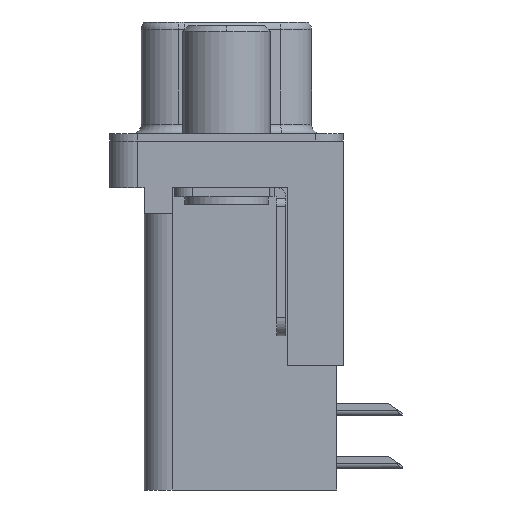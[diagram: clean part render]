
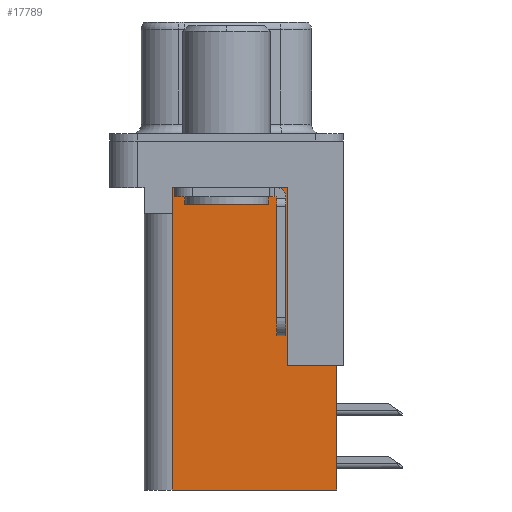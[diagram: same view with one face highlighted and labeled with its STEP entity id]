
A CAD part, left-side view. The second image highlights one B-rep face of the part: STEP entity #17789.
In plain terms, the highlighted planar face has unit normal (-1, 0, 0).
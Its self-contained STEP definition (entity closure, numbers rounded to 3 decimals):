
#487 = VERTEX_POINT ( 'NONE', #7393 ) ;
#774 = LINE ( 'NONE', #2500, #13291 ) ;
#922 = VERTEX_POINT ( 'NONE', #18840 ) ;
#1169 = CARTESIAN_POINT ( 'NONE',  ( 3.765, 2.925, -3.9 ) ) ;
#1815 = EDGE_CURVE ( 'NONE', #922, #18668, #774, .T. ) ;
#1860 = ORIENTED_EDGE ( 'NONE', *, *, #8985, .T. ) ;
#2018 = ORIENTED_EDGE ( 'NONE', *, *, #5487, .F. ) ;
#2265 = CARTESIAN_POINT ( 'NONE',  ( 3.765, 2.925, -18.76 ) ) ;
#2500 = CARTESIAN_POINT ( 'NONE',  ( 3.765, -3.295, -2.5 ) ) ;
#2545 = CARTESIAN_POINT ( 'NONE',  ( 3.765, -3.295, -12.05 ) ) ;
#3403 = EDGE_CURVE ( 'NONE', #17140, #6031, #16879, .T. ) ;
#3794 = AXIS2_PLACEMENT_3D ( 'NONE', #10545, #9117, #19106 ) ;
#4094 = CARTESIAN_POINT ( 'NONE',  ( 3.765, -5.925, -18.76 ) ) ;
#4135 = ORIENTED_EDGE ( 'NONE', *, *, #17022, .F. ) ;
#4360 = VECTOR ( 'NONE', #17735, 1000. ) ;
#4642 = LINE ( 'NONE', #7071, #4360 ) ;
#5293 = LINE ( 'NONE', #15149, #5314 ) ;
#5314 = VECTOR ( 'NONE', #10852, 1000. ) ;
#5487 = EDGE_CURVE ( 'NONE', #487, #17140, #5866, .T. ) ;
#5494 = VERTEX_POINT ( 'NONE', #18474 ) ;
#5577 = EDGE_CURVE ( 'NONE', #487, #15746, #5293, .T. ) ;
#5667 = EDGE_CURVE ( 'NONE', #15746, #922, #4642, .T. ) ;
#5844 = VECTOR ( 'NONE', #13128, 1000. ) ;
#5866 = LINE ( 'NONE', #16478, #5844 ) ;
#6031 = VERTEX_POINT ( 'NONE', #18640 ) ;
#6368 = ORIENTED_EDGE ( 'NONE', *, *, #5667, .T. ) ;
#6706 = ORIENTED_EDGE ( 'NONE', *, *, #9367, .T. ) ;
#6995 = DIRECTION ( 'NONE',  ( 0., 0., 1. ) ) ;
#7071 = CARTESIAN_POINT ( 'NONE',  ( 3.765, -3.295, -18.76 ) ) ;
#7318 = VECTOR ( 'NONE', #14339, 1000. ) ;
#7350 = LINE ( 'NONE', #10540, #7318 ) ;
#7393 = CARTESIAN_POINT ( 'NONE',  ( 3.765, -5.925, -12.05 ) ) ;
#7985 = DIRECTION ( 'NONE',  ( 0., 1., 0. ) ) ;
#8952 = ORIENTED_EDGE ( 'NONE', *, *, #3403, .F. ) ;
#8985 = EDGE_CURVE ( 'NONE', #18668, #5494, #9041, .T. ) ;
#9000 = VECTOR ( 'NONE', #9950, 1000. ) ;
#9041 = LINE ( 'NONE', #9492, #9000 ) ;
#9117 = DIRECTION ( 'NONE',  ( 1., 0., 0. ) ) ;
#9367 = EDGE_CURVE ( 'NONE', #5494, #16487, #7350, .T. ) ;
#9492 = CARTESIAN_POINT ( 'NONE',  ( 3.765, 2.895, -3.9 ) ) ;
#9950 = DIRECTION ( 'NONE',  ( 0., 0., -1. ) ) ;
#10540 = CARTESIAN_POINT ( 'NONE',  ( 3.765, 0., -3.9 ) ) ;
#10545 = CARTESIAN_POINT ( 'NONE',  ( 3.765, -3.295, -18.76 ) ) ;
#10665 = EDGE_LOOP ( 'NONE', ( #12805, #1860, #6706, #4135, #8952, #2018, #11916, #6368 ) ) ;
#10852 = DIRECTION ( 'NONE',  ( 0., 1., 0. ) ) ;
#11916 = ORIENTED_EDGE ( 'NONE', *, *, #5577, .T. ) ;
#12805 = ORIENTED_EDGE ( 'NONE', *, *, #1815, .T. ) ;
#13128 = DIRECTION ( 'NONE',  ( 0., 0., -1. ) ) ;
#13291 = VECTOR ( 'NONE', #14532, 1000. ) ;
#13578 = CARTESIAN_POINT ( 'NONE',  ( 3.765, 2.895, -2.5 ) ) ;
#14339 = DIRECTION ( 'NONE',  ( 0., 1., 0. ) ) ;
#14532 = DIRECTION ( 'NONE',  ( 0., 1., 0. ) ) ;
#15149 = CARTESIAN_POINT ( 'NONE',  ( 3.765, -6.295, -12.05 ) ) ;
#15320 = VECTOR ( 'NONE', #6995, 1000. ) ;
#15341 = LINE ( 'NONE', #2265, #15320 ) ;
#15407 = CARTESIAN_POINT ( 'NONE',  ( 3.765, -3.295, -18.76 ) ) ;
#15746 = VERTEX_POINT ( 'NONE', #2545 ) ;
#16478 = CARTESIAN_POINT ( 'NONE',  ( 3.765, -5.925, -2. ) ) ;
#16487 = VERTEX_POINT ( 'NONE', #1169 ) ;
#16657 = VECTOR ( 'NONE', #7985, 1000. ) ;
#16879 = LINE ( 'NONE', #15407, #16657 ) ;
#17022 = EDGE_CURVE ( 'NONE', #6031, #16487, #15341, .T. ) ;
#17140 = VERTEX_POINT ( 'NONE', #4094 ) ;
#17734 = PLANE ( 'NONE',  #3794 ) ;
#17735 = DIRECTION ( 'NONE',  ( 0., 0., 1. ) ) ;
#17789 = ADVANCED_FACE ( 'NONE', ( #17795 ), #17734, .F. ) ;
#17795 = FACE_OUTER_BOUND ( 'NONE', #10665, .T. ) ;
#18474 = CARTESIAN_POINT ( 'NONE',  ( 3.765, 2.895, -3.9 ) ) ;
#18640 = CARTESIAN_POINT ( 'NONE',  ( 3.765, 2.925, -18.76 ) ) ;
#18668 = VERTEX_POINT ( 'NONE', #13578 ) ;
#18840 = CARTESIAN_POINT ( 'NONE',  ( 3.765, -3.295, -2.5 ) ) ;
#19106 = DIRECTION ( 'NONE',  ( 0., 1., 0. ) ) ;
